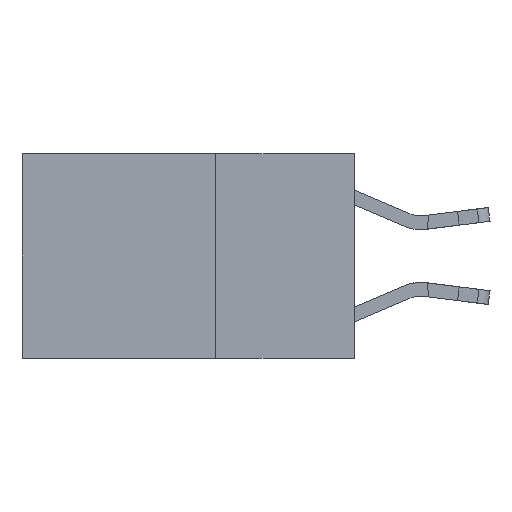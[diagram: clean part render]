
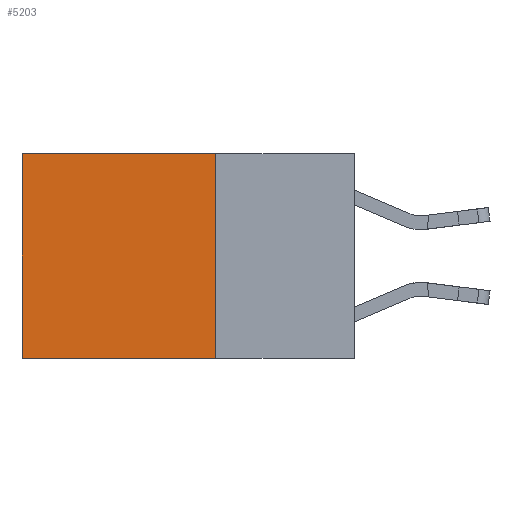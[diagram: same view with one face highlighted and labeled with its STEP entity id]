
A CAD part, left-side view. The second image highlights one B-rep face of the part: STEP entity #5203.
In plain terms, the highlighted planar face has unit normal (-1, 0, 0).
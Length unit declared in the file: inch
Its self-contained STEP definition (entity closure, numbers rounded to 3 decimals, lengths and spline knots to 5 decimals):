
#863 = CARTESIAN_POINT ( 'NONE',  ( 0.2625, 0.25, 0. ) ) ;
#1602 = EDGE_LOOP ( 'NONE', ( #1982, #23201, #14796, #22830 ) ) ;
#1982 = ORIENTED_EDGE ( 'NONE', *, *, #10940, .T. ) ;
#2047 = CARTESIAN_POINT ( 'NONE',  ( 0.2625, 0.6, 0. ) ) ;
#2241 = FACE_OUTER_BOUND ( 'NONE', #1602, .T. ) ;
#2900 = VERTEX_POINT ( 'NONE', #2047 ) ;
#2938 = VECTOR ( 'NONE', #23103, 39.37008 ) ;
#3642 = LINE ( 'NONE', #18968, #2938 ) ;
#3868 = EDGE_CURVE ( 'NONE', #24714, #18449, #7917, .T. ) ;
#4821 = CARTESIAN_POINT ( 'NONE',  ( 0.2625, 0.25, 0. ) ) ;
#4925 = VECTOR ( 'NONE', #24976, 39.37008 ) ;
#5203 = ADVANCED_FACE ( 'NONE', ( #2241 ), #10175, .F. ) ;
#6142 = CARTESIAN_POINT ( 'NONE',  ( 0.2625, 0.25, 0. ) ) ;
#7010 = EDGE_CURVE ( 'NONE', #24128, #2900, #24469, .T. ) ;
#7091 = VECTOR ( 'NONE', #24750, 39.37008 ) ;
#7917 = LINE ( 'NONE', #24875, #25487 ) ;
#8219 = AXIS2_PLACEMENT_3D ( 'NONE', #6142, #17735, #13846 ) ;
#10175 = PLANE ( 'NONE',  #8219 ) ;
#10632 = CARTESIAN_POINT ( 'NONE',  ( 0.2625, 0.6, -0.37 ) ) ;
#10634 = DIRECTION ( 'NONE',  ( 0., 1., 0. ) ) ;
#10940 = EDGE_CURVE ( 'NONE', #2900, #18449, #16639, .T. ) ;
#12052 = CARTESIAN_POINT ( 'NONE',  ( 0.2625, 0.25, -0.37 ) ) ;
#13846 = DIRECTION ( 'NONE',  ( 0., 0., -1. ) ) ;
#14796 = ORIENTED_EDGE ( 'NONE', *, *, #20966, .F. ) ;
#14833 = CARTESIAN_POINT ( 'NONE',  ( 0.2625, 0.6, 0. ) ) ;
#16639 = LINE ( 'NONE', #14833, #7091 ) ;
#17735 = DIRECTION ( 'NONE',  ( 1., 0., 0. ) ) ;
#18449 = VERTEX_POINT ( 'NONE', #10632 ) ;
#18968 = CARTESIAN_POINT ( 'NONE',  ( 0.2625, 0.25, 0. ) ) ;
#20966 = EDGE_CURVE ( 'NONE', #24128, #24714, #3642, .T. ) ;
#22830 = ORIENTED_EDGE ( 'NONE', *, *, #7010, .T. ) ;
#23103 = DIRECTION ( 'NONE',  ( 0., 0., -1. ) ) ;
#23201 = ORIENTED_EDGE ( 'NONE', *, *, #3868, .F. ) ;
#24128 = VERTEX_POINT ( 'NONE', #4821 ) ;
#24469 = LINE ( 'NONE', #863, #4925 ) ;
#24714 = VERTEX_POINT ( 'NONE', #12052 ) ;
#24750 = DIRECTION ( 'NONE',  ( 0., 0., -1. ) ) ;
#24875 = CARTESIAN_POINT ( 'NONE',  ( 0.2625, 0.25, -0.37 ) ) ;
#24976 = DIRECTION ( 'NONE',  ( 0., 1., 0. ) ) ;
#25487 = VECTOR ( 'NONE', #10634, 39.37008 ) ;
